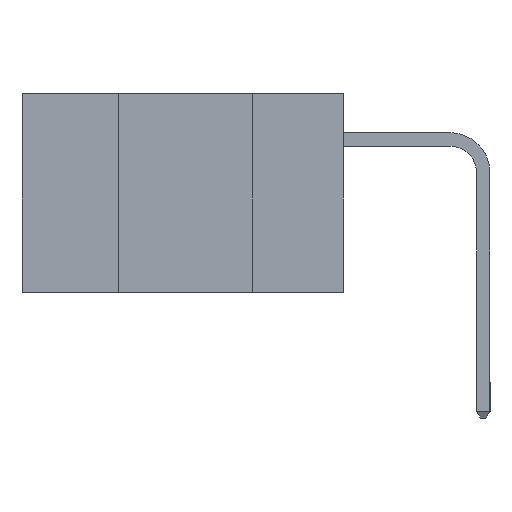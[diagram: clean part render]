
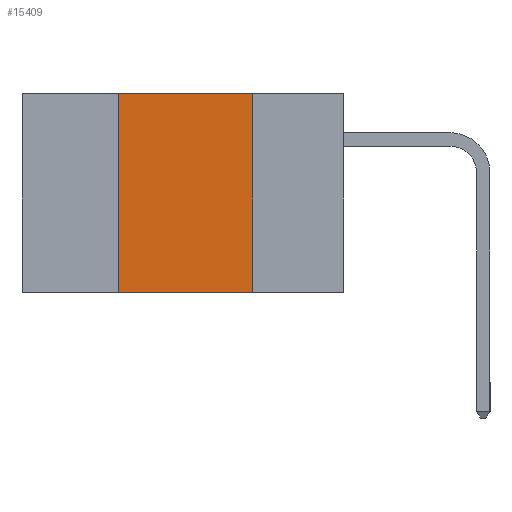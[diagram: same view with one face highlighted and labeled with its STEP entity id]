
A CAD part, left-side view. The second image highlights one B-rep face of the part: STEP entity #15409.
In plain terms, the highlighted planar face has unit normal (-1, 0, 0).
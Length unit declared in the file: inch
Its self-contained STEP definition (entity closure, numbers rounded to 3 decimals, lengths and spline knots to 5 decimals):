
#9 = DIRECTION ( 'NONE',  ( 0., 0., -1. ) ) ;
#731 = VECTOR ( 'NONE', #9, 39.37008 ) ;
#1207 = LINE ( 'NONE', #3159, #9171 ) ;
#1937 = FACE_OUTER_BOUND ( 'NONE', #17222, .T. ) ;
#3159 = CARTESIAN_POINT ( 'NONE',  ( 0., 0.6, 0. ) ) ;
#5029 = LINE ( 'NONE', #14704, #731 ) ;
#5256 = LINE ( 'NONE', #22304, #14290 ) ;
#5529 = EDGE_CURVE ( 'NONE', #9679, #21500, #1207, .T. ) ;
#5652 = ORIENTED_EDGE ( 'NONE', *, *, #5529, .F. ) ;
#5731 = DIRECTION ( 'NONE',  ( 1., 0., 0. ) ) ;
#5847 = PLANE ( 'NONE',  #21093 ) ;
#6813 = ORIENTED_EDGE ( 'NONE', *, *, #8506, .T. ) ;
#7719 = VERTEX_POINT ( 'NONE', #14744 ) ;
#8506 = EDGE_CURVE ( 'NONE', #13886, #7719, #5256, .T. ) ;
#8686 = DIRECTION ( 'NONE',  ( 0., -1., 0. ) ) ;
#9171 = VECTOR ( 'NONE', #8686, 39.37008 ) ;
#9387 = DIRECTION ( 'NONE',  ( 0., 0., 1. ) ) ;
#9417 = CARTESIAN_POINT ( 'NONE',  ( 0., 0.6, 0. ) ) ;
#9679 = VERTEX_POINT ( 'NONE', #17577 ) ;
#11132 = DIRECTION ( 'NONE',  ( 0., -1., 0. ) ) ;
#12560 = CARTESIAN_POINT ( 'NONE',  ( 0., 0.17, 0. ) ) ;
#13195 = DIRECTION ( 'NONE',  ( 0., 0., -1. ) ) ;
#13886 = VERTEX_POINT ( 'NONE', #17132 ) ;
#14290 = VECTOR ( 'NONE', #11132, 39.37008 ) ;
#14704 = CARTESIAN_POINT ( 'NONE',  ( 0., 0.17, -0.37 ) ) ;
#14708 = EDGE_CURVE ( 'NONE', #13886, #9679, #20535, .T. ) ;
#14744 = CARTESIAN_POINT ( 'NONE',  ( 0., 0.17, -0.37 ) ) ;
#14894 = EDGE_CURVE ( 'NONE', #21500, #7719, #5029, .T. ) ;
#15409 = ADVANCED_FACE ( 'NONE', ( #1937 ), #5847, .F. ) ;
#17132 = CARTESIAN_POINT ( 'NONE',  ( 0., 0.42, -0.37 ) ) ;
#17222 = EDGE_LOOP ( 'NONE', ( #18001, #5652, #18285, #6813 ) ) ;
#17577 = CARTESIAN_POINT ( 'NONE',  ( 0., 0.42, 0. ) ) ;
#18001 = ORIENTED_EDGE ( 'NONE', *, *, #14894, .F. ) ;
#18285 = ORIENTED_EDGE ( 'NONE', *, *, #14708, .F. ) ;
#20299 = VECTOR ( 'NONE', #9387, 39.37008 ) ;
#20535 = LINE ( 'NONE', #24081, #20299 ) ;
#21093 = AXIS2_PLACEMENT_3D ( 'NONE', #9417, #5731, #13195 ) ;
#21500 = VERTEX_POINT ( 'NONE', #12560 ) ;
#22304 = CARTESIAN_POINT ( 'NONE',  ( 0., 0.6, -0.37 ) ) ;
#24081 = CARTESIAN_POINT ( 'NONE',  ( 0., 0.42, -0.37 ) ) ;
